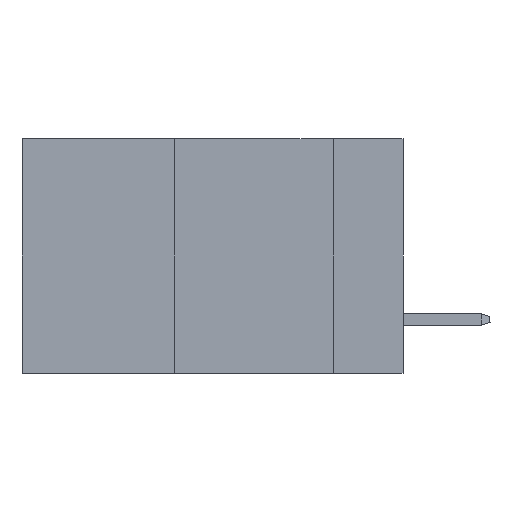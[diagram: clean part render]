
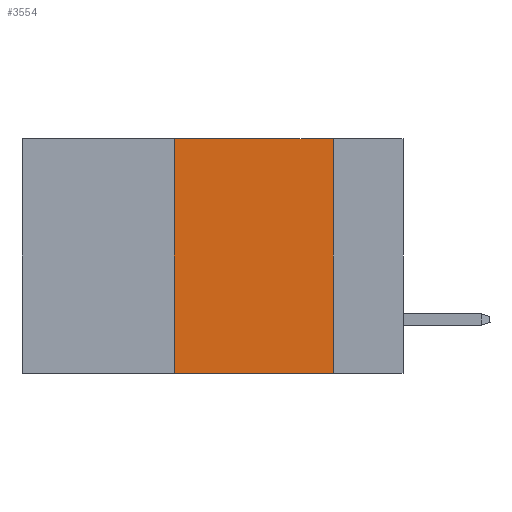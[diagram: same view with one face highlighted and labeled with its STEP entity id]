
A CAD part, left-side view. The second image highlights one B-rep face of the part: STEP entity #3554.
In plain terms, the highlighted planar face has unit normal (-1, 0, 0).
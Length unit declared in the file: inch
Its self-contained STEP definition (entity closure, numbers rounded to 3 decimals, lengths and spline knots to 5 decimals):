
#1751 = LINE ( 'NONE', #2887, #12809 ) ;
#1795 = DIRECTION ( 'NONE',  ( 1., 0., 0. ) ) ;
#2178 = CARTESIAN_POINT ( 'NONE',  ( 0., 0.36, 0. ) ) ;
#2597 = ORIENTED_EDGE ( 'NONE', *, *, #13169, .F. ) ;
#2887 = CARTESIAN_POINT ( 'NONE',  ( 0., 0.6, -0.37 ) ) ;
#3384 = VERTEX_POINT ( 'NONE', #4322 ) ;
#3554 = ADVANCED_FACE ( 'NONE', ( #6422 ), #12645, .F. ) ;
#3594 = AXIS2_PLACEMENT_3D ( 'NONE', #4869, #1795, #14434 ) ;
#4105 = LINE ( 'NONE', #10352, #12537 ) ;
#4322 = CARTESIAN_POINT ( 'NONE',  ( 0., 0.11, 0. ) ) ;
#4708 = VECTOR ( 'NONE', #5270, 39.37008 ) ;
#4840 = VERTEX_POINT ( 'NONE', #5137 ) ;
#4869 = CARTESIAN_POINT ( 'NONE',  ( 0., 0.6, 0. ) ) ;
#5137 = CARTESIAN_POINT ( 'NONE',  ( 0., 0.11, -0.37 ) ) ;
#5222 = VERTEX_POINT ( 'NONE', #16425 ) ;
#5270 = DIRECTION ( 'NONE',  ( 0., 0., 1. ) ) ;
#6309 = EDGE_LOOP ( 'NONE', ( #7873, #14725, #2597, #18569 ) ) ;
#6422 = FACE_OUTER_BOUND ( 'NONE', #6309, .T. ) ;
#6682 = VERTEX_POINT ( 'NONE', #16968 ) ;
#7162 = LINE ( 'NONE', #14786, #13242 ) ;
#7873 = ORIENTED_EDGE ( 'NONE', *, *, #12582, .F. ) ;
#10352 = CARTESIAN_POINT ( 'NONE',  ( 0., 0.11, 0. ) ) ;
#10905 = EDGE_CURVE ( 'NONE', #5222, #4840, #1751, .T. ) ;
#11788 = DIRECTION ( 'NONE',  ( 0., -1., 0. ) ) ;
#12537 = VECTOR ( 'NONE', #16545, 39.37008 ) ;
#12582 = EDGE_CURVE ( 'NONE', #3384, #4840, #4105, .T. ) ;
#12645 = PLANE ( 'NONE',  #3594 ) ;
#12809 = VECTOR ( 'NONE', #20090, 39.37008 ) ;
#13169 = EDGE_CURVE ( 'NONE', #5222, #6682, #16080, .T. ) ;
#13242 = VECTOR ( 'NONE', #11788, 39.37008 ) ;
#14434 = DIRECTION ( 'NONE',  ( 0., 0., -1. ) ) ;
#14725 = ORIENTED_EDGE ( 'NONE', *, *, #16886, .F. ) ;
#14786 = CARTESIAN_POINT ( 'NONE',  ( 0., 0.6, 0. ) ) ;
#16080 = LINE ( 'NONE', #2178, #4708 ) ;
#16425 = CARTESIAN_POINT ( 'NONE',  ( 0., 0.36, -0.37 ) ) ;
#16545 = DIRECTION ( 'NONE',  ( 0., 0., -1. ) ) ;
#16886 = EDGE_CURVE ( 'NONE', #6682, #3384, #7162, .T. ) ;
#16968 = CARTESIAN_POINT ( 'NONE',  ( 0., 0.36, 0. ) ) ;
#18569 = ORIENTED_EDGE ( 'NONE', *, *, #10905, .T. ) ;
#20090 = DIRECTION ( 'NONE',  ( 0., -1., 0. ) ) ;
